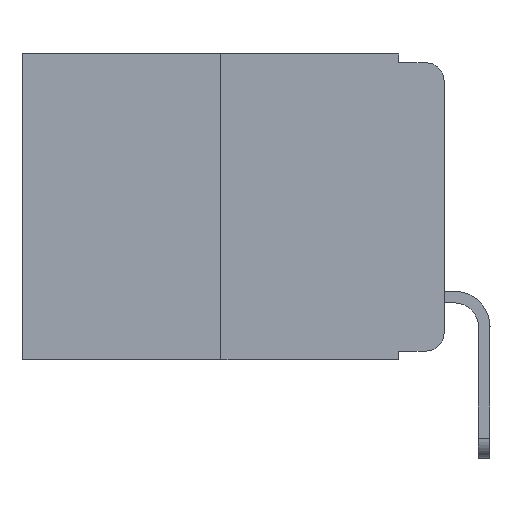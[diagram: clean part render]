
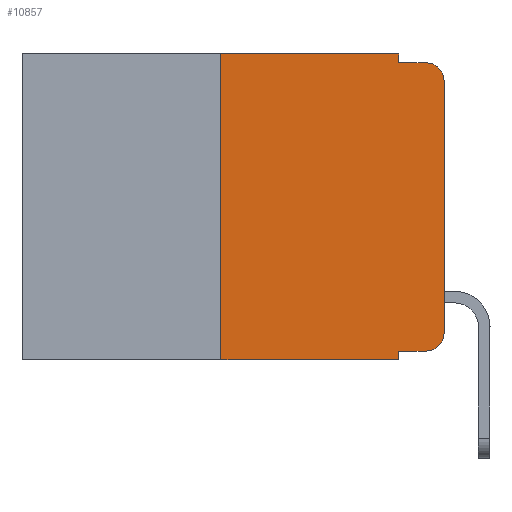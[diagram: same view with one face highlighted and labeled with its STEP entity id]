
A CAD part, left-side view. The second image highlights one B-rep face of the part: STEP entity #10857.
In plain terms, the highlighted planar face has unit normal (-1, 0, 0).
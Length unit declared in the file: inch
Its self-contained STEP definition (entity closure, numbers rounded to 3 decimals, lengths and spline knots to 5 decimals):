
#244 = CIRCLE ( 'NONE', #8894, 0.02 ) ;
#665 = DIRECTION ( 'NONE',  ( 0., 0., 1. ) ) ;
#1108 = DIRECTION ( 'NONE',  ( 0., -1., 0. ) ) ;
#1556 = DIRECTION ( 'NONE',  ( -1., 0., 0. ) ) ;
#1558 = EDGE_CURVE ( 'NONE', #16508, #24189, #1662, .T. ) ;
#1662 = LINE ( 'NONE', #17180, #9383 ) ;
#1746 = CARTESIAN_POINT ( 'NONE',  ( 0., 0.473, 0. ) ) ;
#2102 = ORIENTED_EDGE ( 'NONE', *, *, #7047, .F. ) ;
#2134 = ORIENTED_EDGE ( 'NONE', *, *, #13427, .F. ) ;
#2250 = LINE ( 'NONE', #18268, #12788 ) ;
#4165 = CARTESIAN_POINT ( 'NONE',  ( 0., 0.25, -0.343 ) ) ;
#4172 = ORIENTED_EDGE ( 'NONE', *, *, #11931, .T. ) ;
#4503 = LINE ( 'NONE', #20285, #21554 ) ;
#4742 = DIRECTION ( 'NONE',  ( 0., 0., -1. ) ) ;
#4952 = CARTESIAN_POINT ( 'NONE',  ( 0., 0.02, -0.01 ) ) ;
#5179 = CARTESIAN_POINT ( 'NONE',  ( 0., 0.25, 0. ) ) ;
#5187 = CARTESIAN_POINT ( 'NONE',  ( 0., 0.051, 0. ) ) ;
#5275 = VERTEX_POINT ( 'NONE', #15394 ) ;
#5502 = LINE ( 'NONE', #17787, #7803 ) ;
#5508 = LINE ( 'NONE', #13942, #24818 ) ;
#5617 = ORIENTED_EDGE ( 'NONE', *, *, #17762, .F. ) ;
#5684 = VERTEX_POINT ( 'NONE', #24769 ) ;
#5892 = EDGE_CURVE ( 'NONE', #19284, #23406, #5502, .T. ) ;
#6478 = CARTESIAN_POINT ( 'NONE',  ( 0., 0.051, 0. ) ) ;
#7047 = EDGE_CURVE ( 'NONE', #24189, #5275, #5508, .T. ) ;
#7663 = PLANE ( 'NONE',  #18750 ) ;
#7803 = VECTOR ( 'NONE', #13424, 39.37008 ) ;
#8057 = VECTOR ( 'NONE', #10042, 39.37008 ) ;
#8894 = AXIS2_PLACEMENT_3D ( 'NONE', #24390, #20775, #4742 ) ;
#9383 = VECTOR ( 'NONE', #25054, 39.37008 ) ;
#9667 = DIRECTION ( 'NONE',  ( 0., 0., -1. ) ) ;
#10042 = DIRECTION ( 'NONE',  ( 0., 0., -1. ) ) ;
#10675 = VERTEX_POINT ( 'NONE', #4952 ) ;
#10757 = VERTEX_POINT ( 'NONE', #4165 ) ;
#10857 = ADVANCED_FACE ( 'NONE', ( #11569 ), #7663, .F. ) ;
#10993 = CARTESIAN_POINT ( 'NONE',  ( 0., 0.02, -0.333 ) ) ;
#11446 = ORIENTED_EDGE ( 'NONE', *, *, #12312, .F. ) ;
#11569 = FACE_OUTER_BOUND ( 'NONE', #23692, .T. ) ;
#11576 = EDGE_CURVE ( 'NONE', #23406, #15224, #11769, .T. ) ;
#11701 = DIRECTION ( 'NONE',  ( 1., 0., 0. ) ) ;
#11769 = CIRCLE ( 'NONE', #12195, 0.02 ) ;
#11931 = EDGE_CURVE ( 'NONE', #21898, #10675, #244, .T. ) ;
#11951 = DIRECTION ( 'NONE',  ( 0., 0., -1. ) ) ;
#12129 = CARTESIAN_POINT ( 'NONE',  ( 0., 0., -0.03 ) ) ;
#12195 = AXIS2_PLACEMENT_3D ( 'NONE', #13467, #1556, #15528 ) ;
#12312 = EDGE_CURVE ( 'NONE', #19284, #5684, #20577, .T. ) ;
#12553 = CARTESIAN_POINT ( 'NONE',  ( 0., 0.473, -0.343 ) ) ;
#12788 = VECTOR ( 'NONE', #21886, 39.37008 ) ;
#12869 = CARTESIAN_POINT ( 'NONE',  ( 0., 0.051, -0.01 ) ) ;
#12957 = ORIENTED_EDGE ( 'NONE', *, *, #1558, .F. ) ;
#13424 = DIRECTION ( 'NONE',  ( 0., -1., 0. ) ) ;
#13427 = EDGE_CURVE ( 'NONE', #5275, #10675, #20859, .T. ) ;
#13467 = CARTESIAN_POINT ( 'NONE',  ( 0., 0.02, -0.313 ) ) ;
#13523 = ORIENTED_EDGE ( 'NONE', *, *, #23234, .T. ) ;
#13942 = CARTESIAN_POINT ( 'NONE',  ( 0., 0.051, 0. ) ) ;
#14120 = ORIENTED_EDGE ( 'NONE', *, *, #5892, .T. ) ;
#14370 = DIRECTION ( 'NONE',  ( 0., -1., 0. ) ) ;
#15224 = VERTEX_POINT ( 'NONE', #21609 ) ;
#15394 = CARTESIAN_POINT ( 'NONE',  ( 0., 0.051, -0.01 ) ) ;
#15528 = DIRECTION ( 'NONE',  ( 0., 0., -1. ) ) ;
#16508 = VERTEX_POINT ( 'NONE', #5179 ) ;
#17180 = CARTESIAN_POINT ( 'NONE',  ( 0., 0.473, 0. ) ) ;
#17527 = ORIENTED_EDGE ( 'NONE', *, *, #11576, .T. ) ;
#17762 = EDGE_CURVE ( 'NONE', #10757, #16508, #2250, .T. ) ;
#17787 = CARTESIAN_POINT ( 'NONE',  ( 0., 0.051, -0.333 ) ) ;
#18268 = CARTESIAN_POINT ( 'NONE',  ( 0., 0.25, 0. ) ) ;
#18750 = AXIS2_PLACEMENT_3D ( 'NONE', #1746, #11701, #11951 ) ;
#19284 = VERTEX_POINT ( 'NONE', #24723 ) ;
#19461 = ORIENTED_EDGE ( 'NONE', *, *, #23279, .T. ) ;
#20285 = CARTESIAN_POINT ( 'NONE',  ( 0., 0., 0. ) ) ;
#20577 = LINE ( 'NONE', #6478, #8057 ) ;
#20714 = VECTOR ( 'NONE', #14370, 39.37008 ) ;
#20775 = DIRECTION ( 'NONE',  ( -1., 0., 0. ) ) ;
#20859 = LINE ( 'NONE', #12869, #24987 ) ;
#21554 = VECTOR ( 'NONE', #665, 39.37008 ) ;
#21609 = CARTESIAN_POINT ( 'NONE',  ( 0., 0., -0.313 ) ) ;
#21886 = DIRECTION ( 'NONE',  ( 0., 0., 1. ) ) ;
#21898 = VERTEX_POINT ( 'NONE', #12129 ) ;
#23234 = EDGE_CURVE ( 'NONE', #10757, #5684, #24036, .T. ) ;
#23279 = EDGE_CURVE ( 'NONE', #15224, #21898, #4503, .T. ) ;
#23406 = VERTEX_POINT ( 'NONE', #10993 ) ;
#23692 = EDGE_LOOP ( 'NONE', ( #19461, #4172, #2134, #2102, #12957, #5617, #13523, #11446, #14120, #17527 ) ) ;
#24036 = LINE ( 'NONE', #12553, #20714 ) ;
#24189 = VERTEX_POINT ( 'NONE', #5187 ) ;
#24390 = CARTESIAN_POINT ( 'NONE',  ( 0., 0.02, -0.03 ) ) ;
#24723 = CARTESIAN_POINT ( 'NONE',  ( 0., 0.051, -0.333 ) ) ;
#24769 = CARTESIAN_POINT ( 'NONE',  ( 0., 0.051, -0.343 ) ) ;
#24818 = VECTOR ( 'NONE', #9667, 39.37008 ) ;
#24987 = VECTOR ( 'NONE', #1108, 39.37008 ) ;
#25054 = DIRECTION ( 'NONE',  ( 0., -1., 0. ) ) ;
